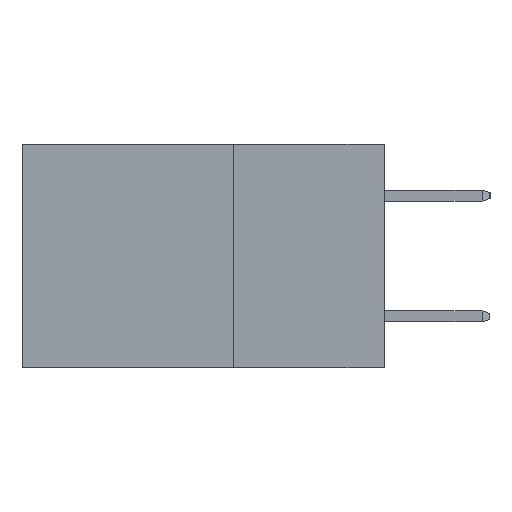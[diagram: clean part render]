
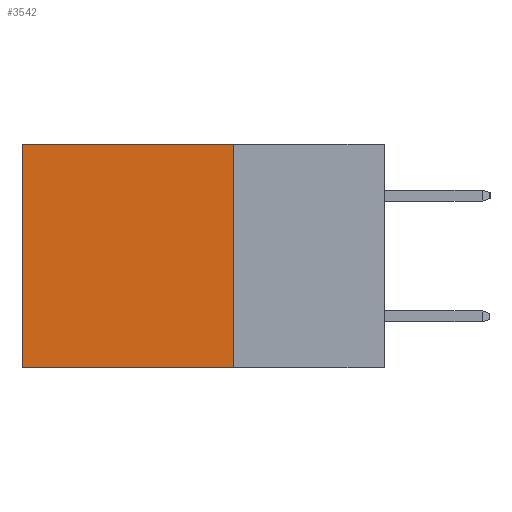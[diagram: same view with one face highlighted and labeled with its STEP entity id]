
A CAD part, left-side view. The second image highlights one B-rep face of the part: STEP entity #3542.
In plain terms, the highlighted planar face has unit normal (-1, 0, 0).
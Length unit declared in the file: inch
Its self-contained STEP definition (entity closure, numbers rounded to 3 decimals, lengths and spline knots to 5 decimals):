
#65 = VECTOR ( 'NONE', #4210, 39.37008 ) ;
#601 = DIRECTION ( 'NONE',  ( 0., 1., 0. ) ) ;
#1013 = VERTEX_POINT ( 'NONE', #3173 ) ;
#1070 = CARTESIAN_POINT ( 'NONE',  ( 0.298, 0.25, 0. ) ) ;
#1133 = PLANE ( 'NONE',  #3147 ) ;
#1206 = CARTESIAN_POINT ( 'NONE',  ( 0.298, 0.25, -0.37 ) ) ;
#1408 = LINE ( 'NONE', #1206, #7576 ) ;
#1828 = CARTESIAN_POINT ( 'NONE',  ( 0.298, 0.6, -0.37 ) ) ;
#1964 = ORIENTED_EDGE ( 'NONE', *, *, #6989, .F. ) ;
#2452 = DIRECTION ( 'NONE',  ( 0., 1., 0. ) ) ;
#2699 = VERTEX_POINT ( 'NONE', #7810 ) ;
#3147 = AXIS2_PLACEMENT_3D ( 'NONE', #1070, #12903, #12852 ) ;
#3173 = CARTESIAN_POINT ( 'NONE',  ( 0.298, 0.25, 0. ) ) ;
#3542 = ADVANCED_FACE ( 'NONE', ( #12548 ), #1133, .F. ) ;
#4066 = ORIENTED_EDGE ( 'NONE', *, *, #5732, .T. ) ;
#4210 = DIRECTION ( 'NONE',  ( 0., 0., -1. ) ) ;
#5081 = VECTOR ( 'NONE', #8453, 39.37008 ) ;
#5184 = CARTESIAN_POINT ( 'NONE',  ( 0.298, 0.6, 0. ) ) ;
#5705 = VERTEX_POINT ( 'NONE', #5184 ) ;
#5732 = EDGE_CURVE ( 'NONE', #1013, #5705, #10309, .T. ) ;
#6250 = VECTOR ( 'NONE', #601, 39.37008 ) ;
#6668 = EDGE_CURVE ( 'NONE', #5705, #8386, #11695, .T. ) ;
#6691 = EDGE_CURVE ( 'NONE', #2699, #8386, #1408, .T. ) ;
#6989 = EDGE_CURVE ( 'NONE', #1013, #2699, #9502, .T. ) ;
#7057 = EDGE_LOOP ( 'NONE', ( #7130, #9611, #1964, #4066 ) ) ;
#7130 = ORIENTED_EDGE ( 'NONE', *, *, #6668, .T. ) ;
#7576 = VECTOR ( 'NONE', #2452, 39.37008 ) ;
#7810 = CARTESIAN_POINT ( 'NONE',  ( 0.298, 0.25, -0.37 ) ) ;
#8386 = VERTEX_POINT ( 'NONE', #1828 ) ;
#8453 = DIRECTION ( 'NONE',  ( 0., 0., -1. ) ) ;
#9502 = LINE ( 'NONE', #11655, #65 ) ;
#9611 = ORIENTED_EDGE ( 'NONE', *, *, #6691, .F. ) ;
#10309 = LINE ( 'NONE', #11241, #6250 ) ;
#11241 = CARTESIAN_POINT ( 'NONE',  ( 0.298, 0.25, 0. ) ) ;
#11655 = CARTESIAN_POINT ( 'NONE',  ( 0.298, 0.25, 0. ) ) ;
#11695 = LINE ( 'NONE', #13463, #5081 ) ;
#12548 = FACE_OUTER_BOUND ( 'NONE', #7057, .T. ) ;
#12852 = DIRECTION ( 'NONE',  ( 0., 0., -1. ) ) ;
#12903 = DIRECTION ( 'NONE',  ( 1., 0., 0. ) ) ;
#13463 = CARTESIAN_POINT ( 'NONE',  ( 0.298, 0.6, 0. ) ) ;
